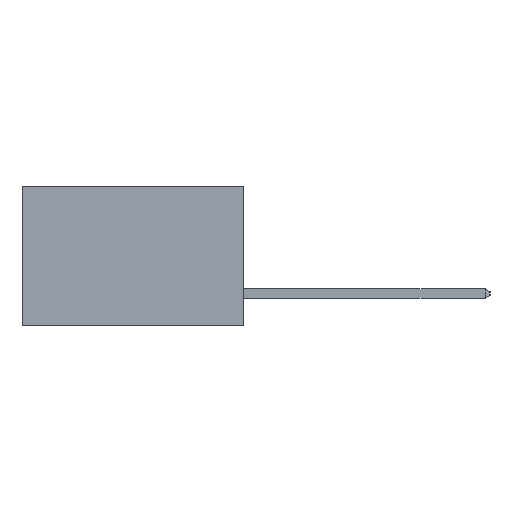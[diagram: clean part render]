
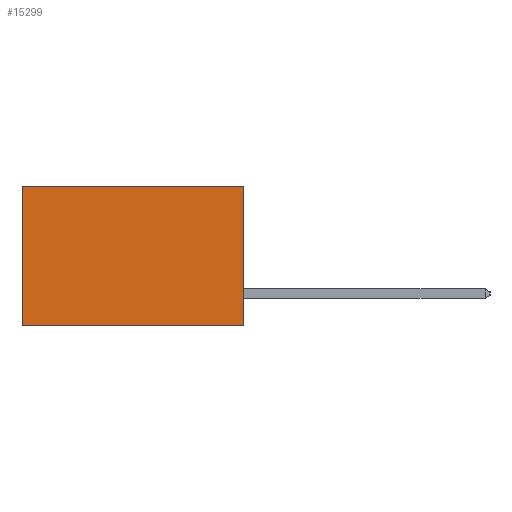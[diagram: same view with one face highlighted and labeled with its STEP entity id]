
A CAD part, left-side view. The second image highlights one B-rep face of the part: STEP entity #15299.
In plain terms, the highlighted planar face has unit normal (-1, 0, 0).
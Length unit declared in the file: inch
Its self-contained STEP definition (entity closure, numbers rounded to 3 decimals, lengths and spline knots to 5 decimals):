
#441 = EDGE_CURVE ( 'NONE', #20309, #8922, #2282, .T. ) ;
#1394 = EDGE_CURVE ( 'NONE', #15623, #8922, #18250, .T. ) ;
#1564 = LINE ( 'NONE', #21548, #10871 ) ;
#2282 = LINE ( 'NONE', #2865, #15780 ) ;
#2391 = ORIENTED_EDGE ( 'NONE', *, *, #441, .T. ) ;
#2855 = AXIS2_PLACEMENT_3D ( 'NONE', #16678, #5740, #18445 ) ;
#2862 = DIRECTION ( 'NONE',  ( 0., 1., 0. ) ) ;
#2865 = CARTESIAN_POINT ( 'NONE',  ( 0.277, 0.59, -0.37 ) ) ;
#3623 = LINE ( 'NONE', #17578, #21735 ) ;
#3875 = PLANE ( 'NONE',  #2855 ) ;
#5740 = DIRECTION ( 'NONE',  ( 1., 0., 0. ) ) ;
#6644 = CARTESIAN_POINT ( 'NONE',  ( 0.277, 0., -0.37 ) ) ;
#7951 = CARTESIAN_POINT ( 'NONE',  ( 0.277, 0.59, -0.37 ) ) ;
#8922 = VERTEX_POINT ( 'NONE', #7951 ) ;
#9116 = DIRECTION ( 'NONE',  ( 0., 0., -1. ) ) ;
#9138 = CARTESIAN_POINT ( 'NONE',  ( 0.277, 0.59, 0. ) ) ;
#10871 = VECTOR ( 'NONE', #9116, 39.37008 ) ;
#12269 = ORIENTED_EDGE ( 'NONE', *, *, #18988, .F. ) ;
#13201 = VERTEX_POINT ( 'NONE', #18255 ) ;
#15114 = DIRECTION ( 'NONE',  ( 0., 0., -1. ) ) ;
#15299 = ADVANCED_FACE ( 'NONE', ( #19147 ), #3875, .F. ) ;
#15623 = VERTEX_POINT ( 'NONE', #6644 ) ;
#15780 = VECTOR ( 'NONE', #15114, 39.37008 ) ;
#15854 = ORIENTED_EDGE ( 'NONE', *, *, #20124, .T. ) ;
#16598 = DIRECTION ( 'NONE',  ( 0., 1., 0. ) ) ;
#16678 = CARTESIAN_POINT ( 'NONE',  ( 0.277, 0., -0.37 ) ) ;
#17578 = CARTESIAN_POINT ( 'NONE',  ( 0.277, 0., 0. ) ) ;
#18250 = LINE ( 'NONE', #19417, #22337 ) ;
#18255 = CARTESIAN_POINT ( 'NONE',  ( 0.277, 0., 0. ) ) ;
#18445 = DIRECTION ( 'NONE',  ( 0., 0., -1. ) ) ;
#18988 = EDGE_CURVE ( 'NONE', #13201, #15623, #1564, .T. ) ;
#19147 = FACE_OUTER_BOUND ( 'NONE', #19836, .T. ) ;
#19417 = CARTESIAN_POINT ( 'NONE',  ( 0.277, 0., -0.37 ) ) ;
#19836 = EDGE_LOOP ( 'NONE', ( #2391, #22450, #12269, #15854 ) ) ;
#20124 = EDGE_CURVE ( 'NONE', #13201, #20309, #3623, .T. ) ;
#20309 = VERTEX_POINT ( 'NONE', #9138 ) ;
#21548 = CARTESIAN_POINT ( 'NONE',  ( 0.277, 0., -0.37 ) ) ;
#21735 = VECTOR ( 'NONE', #2862, 39.37008 ) ;
#22337 = VECTOR ( 'NONE', #16598, 39.37008 ) ;
#22450 = ORIENTED_EDGE ( 'NONE', *, *, #1394, .F. ) ;
